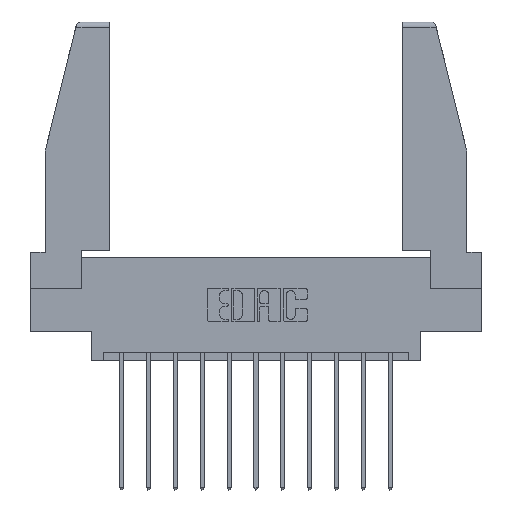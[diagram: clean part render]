
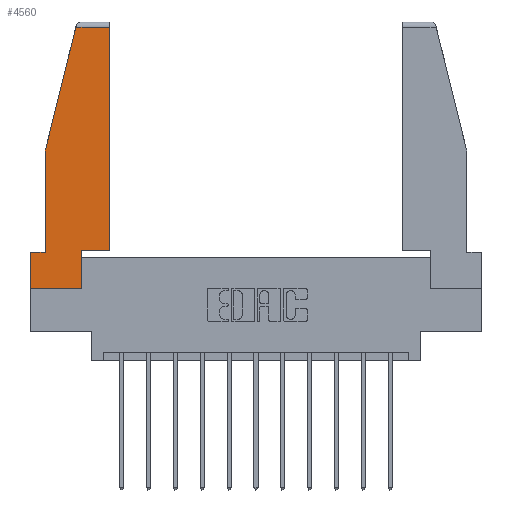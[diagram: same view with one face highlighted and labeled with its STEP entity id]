
A CAD part, top view. The second image highlights one B-rep face of the part: STEP entity #4560.
In plain terms, the highlighted planar face has unit normal (0, 0, 1).
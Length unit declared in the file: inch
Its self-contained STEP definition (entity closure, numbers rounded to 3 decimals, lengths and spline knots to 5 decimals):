
#223 = ORIENTED_EDGE ( 'NONE', *, *, #6050, .T. ) ;
#291 = CARTESIAN_POINT ( 'NONE',  ( 0., 0., 0. ) ) ;
#404 = CARTESIAN_POINT ( 'NONE',  ( 0.271, 1.55, 0. ) ) ;
#515 = VERTEX_POINT ( 'NONE', #6717 ) ;
#559 = VECTOR ( 'NONE', #8454, 39.37008 ) ;
#688 = VERTEX_POINT ( 'NONE', #3906 ) ;
#812 = VECTOR ( 'NONE', #3300, 39.37008 ) ;
#1282 = CARTESIAN_POINT ( 'NONE',  ( 0.297, 0.223, 0. ) ) ;
#1762 = VECTOR ( 'NONE', #15106, 39.37008 ) ;
#1891 = VECTOR ( 'NONE', #11397, 39.37008 ) ;
#1909 = VECTOR ( 'NONE', #7849, 39.37008 ) ;
#1992 = ORIENTED_EDGE ( 'NONE', *, *, #10148, .T. ) ;
#2152 = DIRECTION ( 'NONE',  ( -1., 0., 0. ) ) ;
#2220 = PLANE ( 'NONE',  #6639 ) ;
#2522 = ORIENTED_EDGE ( 'NONE', *, *, #7424, .T. ) ;
#2682 = EDGE_CURVE ( 'NONE', #688, #13152, #11611, .T. ) ;
#2772 = VECTOR ( 'NONE', #10737, 39.37008 ) ;
#2885 = ORIENTED_EDGE ( 'NONE', *, *, #8517, .T. ) ;
#3145 = FACE_OUTER_BOUND ( 'NONE', #14382, .T. ) ;
#3300 = DIRECTION ( 'NONE',  ( 0., 1., 0. ) ) ;
#3484 = VECTOR ( 'NONE', #14656, 39.37008 ) ;
#3621 = CARTESIAN_POINT ( 'NONE',  ( 0.2636, 1.52, 0. ) ) ;
#3678 = CARTESIAN_POINT ( 'NONE',  ( 0., 0.21, 0. ) ) ;
#3778 = DIRECTION ( 'NONE',  ( -0.239, -0.971, 0. ) ) ;
#3906 = CARTESIAN_POINT ( 'NONE',  ( 0.086, 0.8, 0. ) ) ;
#3942 = VECTOR ( 'NONE', #2152, 39.37008 ) ;
#4035 = ORIENTED_EDGE ( 'NONE', *, *, #7012, .T. ) ;
#4189 = VERTEX_POINT ( 'NONE', #11160 ) ;
#4560 = ADVANCED_FACE ( 'NONE', ( #3145 ), #2220, .T. ) ;
#4610 = CARTESIAN_POINT ( 'NONE',  ( 0.297, 0., 0. ) ) ;
#5466 = CARTESIAN_POINT ( 'NONE',  ( 0.086, 0.8, 0. ) ) ;
#5983 = ORIENTED_EDGE ( 'NONE', *, *, #9743, .T. ) ;
#6050 = EDGE_CURVE ( 'NONE', #10616, #4189, #7994, .T. ) ;
#6066 = CARTESIAN_POINT ( 'NONE',  ( 0.461, 0.223, 0. ) ) ;
#6639 = AXIS2_PLACEMENT_3D ( 'NONE', #10207, #7950, #7999 ) ;
#6680 = LINE ( 'NONE', #9099, #3942 ) ;
#6717 = CARTESIAN_POINT ( 'NONE',  ( 0.461, 1.52, 0. ) ) ;
#7012 = EDGE_CURVE ( 'NONE', #515, #13305, #6680, .T. ) ;
#7066 = EDGE_CURVE ( 'NONE', #10325, #515, #9801, .T. ) ;
#7340 = ORIENTED_EDGE ( 'NONE', *, *, #7066, .T. ) ;
#7424 = EDGE_CURVE ( 'NONE', #13152, #11379, #10527, .T. ) ;
#7747 = CARTESIAN_POINT ( 'NONE',  ( 0.297, 0., 0. ) ) ;
#7849 = DIRECTION ( 'NONE',  ( -1., 0., 0. ) ) ;
#7950 = DIRECTION ( 'NONE',  ( 0., 0., 1. ) ) ;
#7994 = LINE ( 'NONE', #4610, #1762 ) ;
#7999 = DIRECTION ( 'NONE',  ( 1., 0., 0. ) ) ;
#8454 = DIRECTION ( 'NONE',  ( 1., 0., 0. ) ) ;
#8517 = EDGE_CURVE ( 'NONE', #13305, #688, #11032, .T. ) ;
#8665 = ORIENTED_EDGE ( 'NONE', *, *, #13052, .T. ) ;
#9099 = CARTESIAN_POINT ( 'NONE',  ( 0., 1.52, 0. ) ) ;
#9743 = EDGE_CURVE ( 'NONE', #4189, #10325, #13738, .T. ) ;
#9801 = LINE ( 'NONE', #14991, #812 ) ;
#10083 = VERTEX_POINT ( 'NONE', #291 ) ;
#10148 = EDGE_CURVE ( 'NONE', #11379, #10083, #14103, .T. ) ;
#10207 = CARTESIAN_POINT ( 'NONE',  ( 0., 0., 0. ) ) ;
#10325 = VERTEX_POINT ( 'NONE', #6066 ) ;
#10527 = LINE ( 'NONE', #11378, #1909 ) ;
#10616 = VERTEX_POINT ( 'NONE', #7747 ) ;
#10628 = CARTESIAN_POINT ( 'NONE',  ( 0.086, 0.21, 0. ) ) ;
#10737 = DIRECTION ( 'NONE',  ( 0., -1., 0. ) ) ;
#11032 = LINE ( 'NONE', #404, #13780 ) ;
#11160 = CARTESIAN_POINT ( 'NONE',  ( 0.297, 0.223, 0. ) ) ;
#11378 = CARTESIAN_POINT ( 'NONE',  ( 0., 0.21, 0. ) ) ;
#11379 = VERTEX_POINT ( 'NONE', #13978 ) ;
#11397 = DIRECTION ( 'NONE',  ( 0., -1., 0. ) ) ;
#11611 = LINE ( 'NONE', #5466, #1891 ) ;
#13052 = EDGE_CURVE ( 'NONE', #10083, #10616, #15014, .T. ) ;
#13152 = VERTEX_POINT ( 'NONE', #10628 ) ;
#13305 = VERTEX_POINT ( 'NONE', #3621 ) ;
#13738 = LINE ( 'NONE', #1282, #559 ) ;
#13780 = VECTOR ( 'NONE', #3778, 39.37008 ) ;
#13934 = ORIENTED_EDGE ( 'NONE', *, *, #2682, .T. ) ;
#13978 = CARTESIAN_POINT ( 'NONE',  ( 0., 0.21, 0. ) ) ;
#14103 = LINE ( 'NONE', #3678, #2772 ) ;
#14340 = CARTESIAN_POINT ( 'NONE',  ( 0., 0., 0. ) ) ;
#14382 = EDGE_LOOP ( 'NONE', ( #7340, #4035, #2885, #13934, #2522, #1992, #8665, #223, #5983 ) ) ;
#14656 = DIRECTION ( 'NONE',  ( 1., 0., 0. ) ) ;
#14991 = CARTESIAN_POINT ( 'NONE',  ( 0.461, 0.223, 0. ) ) ;
#15014 = LINE ( 'NONE', #14340, #3484 ) ;
#15106 = DIRECTION ( 'NONE',  ( 0., 1., 0. ) ) ;
